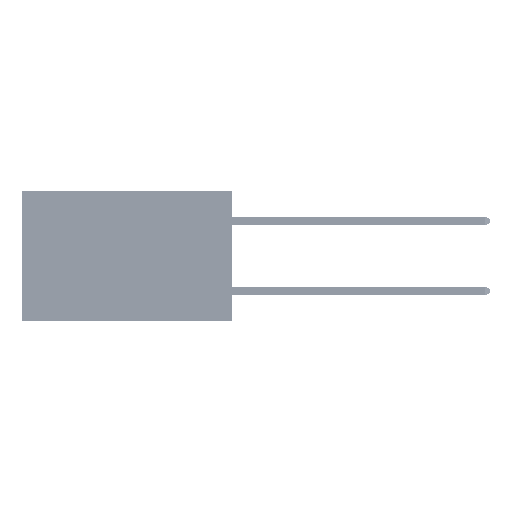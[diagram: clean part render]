
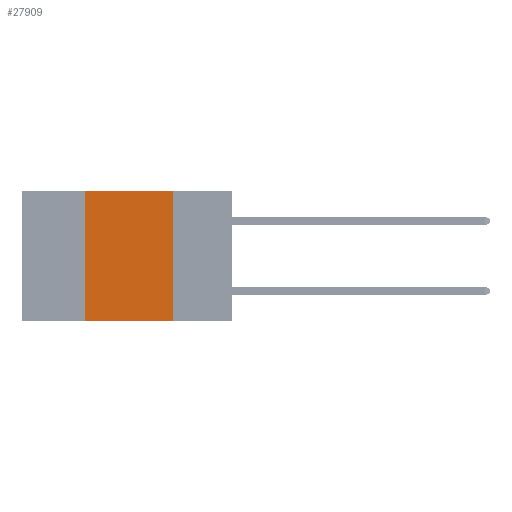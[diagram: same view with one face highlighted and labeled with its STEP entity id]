
A CAD part, left-side view. The second image highlights one B-rep face of the part: STEP entity #27909.
In plain terms, the highlighted planar face has unit normal (-1, 0, 0).
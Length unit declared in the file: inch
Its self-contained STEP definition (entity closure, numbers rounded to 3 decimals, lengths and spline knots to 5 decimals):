
#828 = ORIENTED_EDGE ( 'NONE', *, *, #30737, .F. ) ;
#1205 = LINE ( 'NONE', #23516, #43883 ) ;
#1265 = ORIENTED_EDGE ( 'NONE', *, *, #42550, .F. ) ;
#1432 = ORIENTED_EDGE ( 'NONE', *, *, #24122, .F. ) ;
#1857 = VERTEX_POINT ( 'NONE', #21582 ) ;
#2003 = CARTESIAN_POINT ( 'NONE',  ( 0., 0.6, 0. ) ) ;
#2368 = VERTEX_POINT ( 'NONE', #43059 ) ;
#2461 = EDGE_LOOP ( 'NONE', ( #1265, #1432, #828, #30785 ) ) ;
#5724 = DIRECTION ( 'NONE',  ( 0., -1., 0. ) ) ;
#8339 = VECTOR ( 'NONE', #5724, 39.37008 ) ;
#10566 = EDGE_CURVE ( 'NONE', #2368, #36798, #47751, .T. ) ;
#14004 = VECTOR ( 'NONE', #47180, 39.37008 ) ;
#15446 = FACE_OUTER_BOUND ( 'NONE', #2461, .T. ) ;
#15855 = CARTESIAN_POINT ( 'NONE',  ( 0., 0.42, 0. ) ) ;
#18418 = DIRECTION ( 'NONE',  ( 1., 0., 0. ) ) ;
#19624 = LINE ( 'NONE', #15855, #14004 ) ;
#21582 = CARTESIAN_POINT ( 'NONE',  ( 0., 0.42, 0. ) ) ;
#21675 = CARTESIAN_POINT ( 'NONE',  ( 0., 0.17, -0.37 ) ) ;
#23516 = CARTESIAN_POINT ( 'NONE',  ( 0., 0.6, 0. ) ) ;
#24122 = EDGE_CURVE ( 'NONE', #1857, #33793, #1205, .T. ) ;
#27534 = DIRECTION ( 'NONE',  ( 0., -1., 0. ) ) ;
#27909 = ADVANCED_FACE ( 'NONE', ( #15446 ), #45739, .F. ) ;
#28263 = AXIS2_PLACEMENT_3D ( 'NONE', #2003, #18418, #38046 ) ;
#30737 = EDGE_CURVE ( 'NONE', #2368, #1857, #19624, .T. ) ;
#30785 = ORIENTED_EDGE ( 'NONE', *, *, #10566, .T. ) ;
#31099 = LINE ( 'NONE', #32335, #39859 ) ;
#32335 = CARTESIAN_POINT ( 'NONE',  ( 0., 0.17, 0. ) ) ;
#33793 = VERTEX_POINT ( 'NONE', #42312 ) ;
#36798 = VERTEX_POINT ( 'NONE', #21675 ) ;
#37720 = CARTESIAN_POINT ( 'NONE',  ( 0., 0.6, -0.37 ) ) ;
#38046 = DIRECTION ( 'NONE',  ( 0., 0., -1. ) ) ;
#39859 = VECTOR ( 'NONE', #43998, 39.37008 ) ;
#42312 = CARTESIAN_POINT ( 'NONE',  ( 0., 0.17, 0. ) ) ;
#42550 = EDGE_CURVE ( 'NONE', #33793, #36798, #31099, .T. ) ;
#43059 = CARTESIAN_POINT ( 'NONE',  ( 0., 0.42, -0.37 ) ) ;
#43883 = VECTOR ( 'NONE', #27534, 39.37008 ) ;
#43998 = DIRECTION ( 'NONE',  ( 0., 0., -1. ) ) ;
#45739 = PLANE ( 'NONE',  #28263 ) ;
#47180 = DIRECTION ( 'NONE',  ( 0., 0., 1. ) ) ;
#47751 = LINE ( 'NONE', #37720, #8339 ) ;
